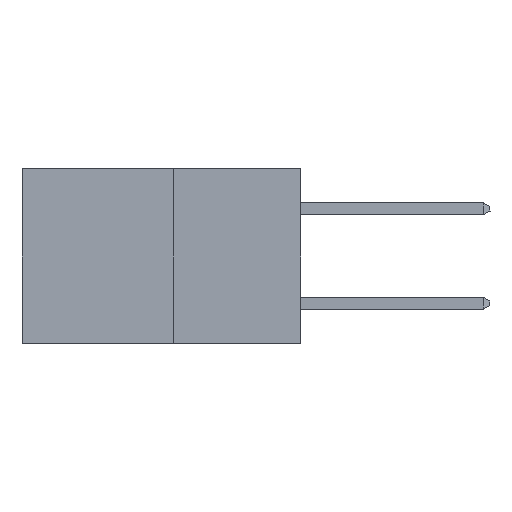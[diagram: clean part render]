
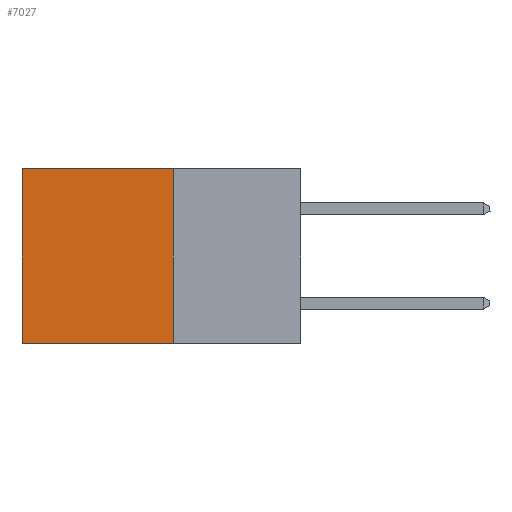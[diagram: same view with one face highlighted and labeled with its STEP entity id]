
A CAD part, left-side view. The second image highlights one B-rep face of the part: STEP entity #7027.
In plain terms, the highlighted planar face has unit normal (-1, 0, 0).
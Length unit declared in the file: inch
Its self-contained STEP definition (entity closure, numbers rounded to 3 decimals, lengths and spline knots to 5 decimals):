
#90 = CARTESIAN_POINT ( 'NONE',  ( 0.277, 0.59, 0. ) ) ;
#458 = VERTEX_POINT ( 'NONE', #20333 ) ;
#539 = VECTOR ( 'NONE', #19623, 39.37008 ) ;
#721 = VECTOR ( 'NONE', #23581, 39.37008 ) ;
#1366 = ORIENTED_EDGE ( 'NONE', *, *, #7974, .F. ) ;
#2463 = VERTEX_POINT ( 'NONE', #90 ) ;
#3474 = ORIENTED_EDGE ( 'NONE', *, *, #23198, .F. ) ;
#4268 = EDGE_CURVE ( 'NONE', #15395, #2463, #8544, .T. ) ;
#7027 = ADVANCED_FACE ( 'NONE', ( #8357 ), #10827, .F. ) ;
#7974 = EDGE_CURVE ( 'NONE', #15395, #458, #8292, .T. ) ;
#8292 = LINE ( 'NONE', #24099, #721 ) ;
#8357 = FACE_OUTER_BOUND ( 'NONE', #25212, .T. ) ;
#8470 = VERTEX_POINT ( 'NONE', #30695 ) ;
#8544 = LINE ( 'NONE', #29354, #15332 ) ;
#10595 = DIRECTION ( 'NONE',  ( 0., 0., -1. ) ) ;
#10760 = DIRECTION ( 'NONE',  ( 1., 0., 0. ) ) ;
#10784 = CARTESIAN_POINT ( 'NONE',  ( 0.277, 0.27, -0.37 ) ) ;
#10827 = PLANE ( 'NONE',  #32000 ) ;
#13264 = ORIENTED_EDGE ( 'NONE', *, *, #4268, .T. ) ;
#15332 = VECTOR ( 'NONE', #29315, 39.37008 ) ;
#15395 = VERTEX_POINT ( 'NONE', #29874 ) ;
#17059 = CARTESIAN_POINT ( 'NONE',  ( 0.277, 0.59, -0.37 ) ) ;
#19623 = DIRECTION ( 'NONE',  ( 0., 0., -1. ) ) ;
#20333 = CARTESIAN_POINT ( 'NONE',  ( 0.277, 0.27, -0.37 ) ) ;
#20886 = LINE ( 'NONE', #17059, #539 ) ;
#21857 = ORIENTED_EDGE ( 'NONE', *, *, #28460, .T. ) ;
#23198 = EDGE_CURVE ( 'NONE', #458, #8470, #27228, .T. ) ;
#23581 = DIRECTION ( 'NONE',  ( 0., 0., -1. ) ) ;
#24099 = CARTESIAN_POINT ( 'NONE',  ( 0.277, 0.27, -0.37 ) ) ;
#25212 = EDGE_LOOP ( 'NONE', ( #21857, #3474, #1366, #13264 ) ) ;
#25660 = VECTOR ( 'NONE', #30068, 39.37008 ) ;
#27228 = LINE ( 'NONE', #27549, #25660 ) ;
#27549 = CARTESIAN_POINT ( 'NONE',  ( 0.277, 0.27, -0.37 ) ) ;
#28460 = EDGE_CURVE ( 'NONE', #2463, #8470, #20886, .T. ) ;
#29315 = DIRECTION ( 'NONE',  ( 0., 1., 0. ) ) ;
#29354 = CARTESIAN_POINT ( 'NONE',  ( 0.277, 0.27, 0. ) ) ;
#29874 = CARTESIAN_POINT ( 'NONE',  ( 0.277, 0.27, 0. ) ) ;
#30068 = DIRECTION ( 'NONE',  ( 0., 1., 0. ) ) ;
#30695 = CARTESIAN_POINT ( 'NONE',  ( 0.277, 0.59, -0.37 ) ) ;
#32000 = AXIS2_PLACEMENT_3D ( 'NONE', #10784, #10760, #10595 ) ;
